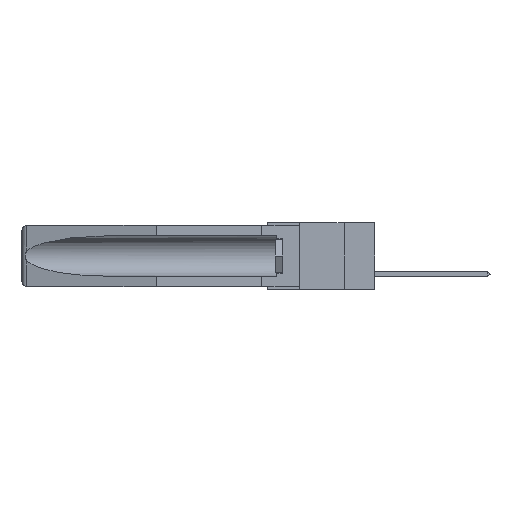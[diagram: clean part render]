
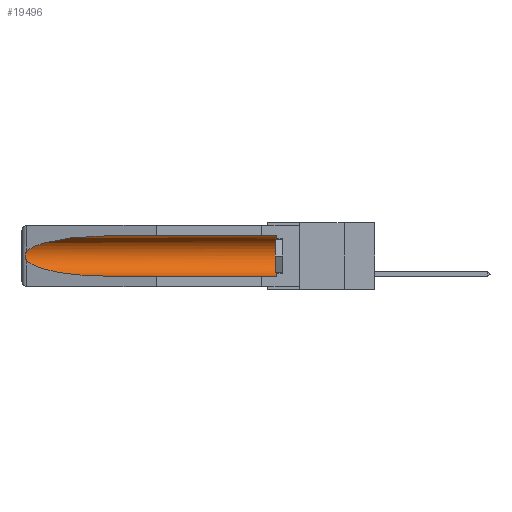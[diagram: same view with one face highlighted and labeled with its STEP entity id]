
A CAD part, left-side view. The second image highlights one B-rep face of the part: STEP entity #19496.
In plain terms, the highlighted cylindrical face has radius 2.857 mm (diameter 5.715 mm), a partial arc.
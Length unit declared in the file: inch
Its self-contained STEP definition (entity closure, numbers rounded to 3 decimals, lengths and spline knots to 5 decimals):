
#2104 = CARTESIAN_POINT ( 'NONE',  ( 0.26537, 1.52718, -0.19328 ) ) ;
#2416 = VERTEX_POINT ( 'NONE', #20471 ) ;
#2771 = CYLINDRICAL_SURFACE ( 'NONE', #8401, 0.1125 ) ;
#2894 = CARTESIAN_POINT ( 'NONE',  ( 0.26654, 1.53092, -0.15636 ) ) ;
#3580 = CARTESIAN_POINT ( 'NONE',  ( 0.155, 0.126, -0.059 ) ) ;
#3780 = DIRECTION ( 'NONE',  ( 0., 1., 0. ) ) ;
#4721 = CARTESIAN_POINT ( 'NONE',  ( 0.26537, 1.52718, -0.19328 ) ) ;
#4887 = ORIENTED_EDGE ( 'NONE', *, *, #14483, .T. ) ;
#5260 = CARTESIAN_POINT ( 'NONE',  ( 0.2675, 1.53308, -0.17534 ) ) ;
#5645 = EDGE_CURVE ( 'NONE', #2416, #25008, #21495, .T. ) ;
#5729 = CARTESIAN_POINT ( 'NONE',  ( 0.26537, 1.52718, -0.14972 ) ) ;
#5932 = CARTESIAN_POINT ( 'NONE',  ( 0.155, -0.30754, -0.1715 ) ) ;
#6129 = DIRECTION ( 'NONE',  ( 0., 0., 1. ) ) ;
#7507 = LINE ( 'NONE', #22789, #13509 ) ;
#7945 = CARTESIAN_POINT ( 'NONE',  ( 0.26537, 1.52718, -0.14972 ) ) ;
#8401 = AXIS2_PLACEMENT_3D ( 'NONE', #5932, #21216, #18576 ) ;
#9652 = B_SPLINE_CURVE_WITH_KNOTS ( 'NONE', 3,
 ( #7945, #20570, #2894, #28084, #30999, #5260, #30531, #20784, #17916, #20349 ),
 .UNSPECIFIED., .F., .F.,
 ( 4, 2, 2, 2, 4 ),
 ( 0., 0.00029, 0.00058, 0.00087, 0.00117 ),
 .UNSPECIFIED. ) ;
#9961 = CARTESIAN_POINT ( 'NONE',  ( 0.21114, 1.30732, -0.284 ) ) ;
#10114 = VERTEX_POINT ( 'NONE', #3580 ) ;
#10710 = EDGE_CURVE ( 'NONE', #16359, #12806, #7507, .T. ) ;
#11878 = CIRCLE ( 'NONE', #24160, 0.1125 ) ;
#11991 = FACE_OUTER_BOUND ( 'NONE', #19509, .T. ) ;
#12075 = EDGE_CURVE ( 'NONE', #31087, #12806, #26051, .T. ) ;
#12806 = VERTEX_POINT ( 'NONE', #22662 ) ;
#13509 = VECTOR ( 'NONE', #27951, 39.37008 ) ;
#14483 = EDGE_CURVE ( 'NONE', #10114, #2416, #18825, .T. ) ;
#14872 = CARTESIAN_POINT ( 'NONE',  ( 0.155, 1.07973, -0.284 ) ) ;
#14986 = CARTESIAN_POINT ( 'NONE',  ( 0.25451, 1.48313, -0.24835 ) ) ;
#16359 = VERTEX_POINT ( 'NONE', #22249 ) ;
#16534 = CARTESIAN_POINT ( 'NONE',  ( 0.155, -0.30754, -0.059 ) ) ;
#16890 = ORIENTED_EDGE ( 'NONE', *, *, #5645, .T. ) ;
#17686 = CARTESIAN_POINT ( 'NONE',  ( 0.25451, 1.48313, -0.09465 ) ) ;
#17916 = CARTESIAN_POINT ( 'NONE',  ( 0.26597, 1.5296, -0.19026 ) ) ;
#18434 = VECTOR ( 'NONE', #3780, 39.37008 ) ;
#18576 = DIRECTION ( 'NONE',  ( 0., 0., 1. ) ) ;
#18825 = LINE ( 'NONE', #16534, #18434 ) ;
#19496 = ADVANCED_FACE ( 'NONE', ( #11991 ), #2771, .F. ) ;
#19509 = EDGE_LOOP ( 'NONE', ( #16890, #30886, #27622, #25021, #29082, #4887 ) ) ;
#20349 = CARTESIAN_POINT ( 'NONE',  ( 0.26537, 1.52718, -0.19328 ) ) ;
#20471 = CARTESIAN_POINT ( 'NONE',  ( 0.155, 1.07973, -0.059 ) ) ;
#20480 = EDGE_CURVE ( 'NONE', #25008, #31087, #9652, .T. ) ;
#20570 = CARTESIAN_POINT ( 'NONE',  ( 0.26597, 1.52961, -0.15275 ) ) ;
#20784 = CARTESIAN_POINT ( 'NONE',  ( 0.26655, 1.53094, -0.18657 ) ) ;
#21216 = DIRECTION ( 'NONE',  ( 0., 1., 0. ) ) ;
#21425 = CARTESIAN_POINT ( 'NONE',  ( 0.155, 0.126, -0.1715 ) ) ;
#21495 =( BOUNDED_CURVE ( )  B_SPLINE_CURVE ( 3, ( #25496, #25149, #17686, #27859 ),
 .UNSPECIFIED., .F., .T. ) 
 B_SPLINE_CURVE_WITH_KNOTS ( ( 4, 4 ),
 ( 4.71239, 6.08839 ),
 .UNSPECIFIED. ) 
 CURVE ( )  GEOMETRIC_REPRESENTATION_ITEM ( )  RATIONAL_B_SPLINE_CURVE ( ( 1., 0.848, 0.848, 1. ) ) 
 REPRESENTATION_ITEM ( '' )  );
#22249 = CARTESIAN_POINT ( 'NONE',  ( 0.155, 0.126, -0.284 ) ) ;
#22662 = CARTESIAN_POINT ( 'NONE',  ( 0.155, 1.07973, -0.284 ) ) ;
#22789 = CARTESIAN_POINT ( 'NONE',  ( 0.155, -0.30754, -0.284 ) ) ;
#23486 = EDGE_CURVE ( 'NONE', #16359, #10114, #11878, .T. ) ;
#24160 = AXIS2_PLACEMENT_3D ( 'NONE', #21425, #28731, #6129 ) ;
#25008 = VERTEX_POINT ( 'NONE', #5729 ) ;
#25021 = ORIENTED_EDGE ( 'NONE', *, *, #10710, .F. ) ;
#25149 = CARTESIAN_POINT ( 'NONE',  ( 0.21114, 1.30732, -0.059 ) ) ;
#25496 = CARTESIAN_POINT ( 'NONE',  ( 0.155, 1.07973, -0.059 ) ) ;
#26051 =( BOUNDED_CURVE ( )  B_SPLINE_CURVE ( 3, ( #2104, #14986, #9961, #14872 ),
 .UNSPECIFIED., .F., .T. ) 
 B_SPLINE_CURVE_WITH_KNOTS ( ( 4, 4 ),
 ( 0.1948, 1.5708 ),
 .UNSPECIFIED. ) 
 CURVE ( )  GEOMETRIC_REPRESENTATION_ITEM ( )  RATIONAL_B_SPLINE_CURVE ( ( 1., 0.848, 0.848, 1. ) ) 
 REPRESENTATION_ITEM ( '' )  );
#27622 = ORIENTED_EDGE ( 'NONE', *, *, #12075, .T. ) ;
#27859 = CARTESIAN_POINT ( 'NONE',  ( 0.26537, 1.52718, -0.14972 ) ) ;
#27951 = DIRECTION ( 'NONE',  ( 0., 1., 0. ) ) ;
#28084 = CARTESIAN_POINT ( 'NONE',  ( 0.2673, 1.5327, -0.16383 ) ) ;
#28731 = DIRECTION ( 'NONE',  ( 0., -1., 0. ) ) ;
#29082 = ORIENTED_EDGE ( 'NONE', *, *, #23486, .T. ) ;
#30531 = CARTESIAN_POINT ( 'NONE',  ( 0.2673, 1.53269, -0.17917 ) ) ;
#30886 = ORIENTED_EDGE ( 'NONE', *, *, #20480, .T. ) ;
#30999 = CARTESIAN_POINT ( 'NONE',  ( 0.2675, 1.53308, -0.16763 ) ) ;
#31087 = VERTEX_POINT ( 'NONE', #4721 ) ;
